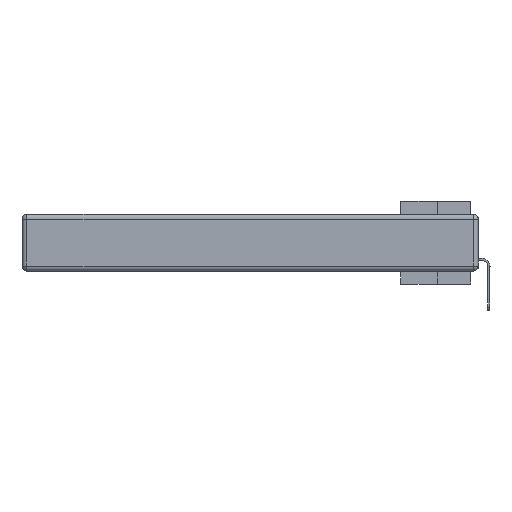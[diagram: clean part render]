
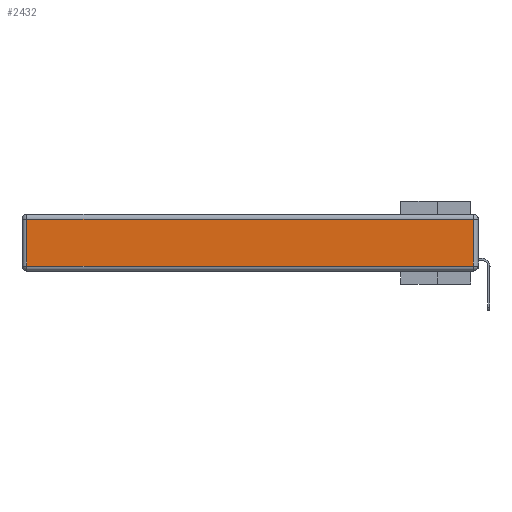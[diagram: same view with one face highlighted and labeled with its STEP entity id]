
A CAD part, left-side view. The second image highlights one B-rep face of the part: STEP entity #2432.
In plain terms, the highlighted planar face has unit normal (-1, 0, 0).
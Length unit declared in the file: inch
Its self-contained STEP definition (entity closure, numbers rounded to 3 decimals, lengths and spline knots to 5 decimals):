
#1082 = EDGE_CURVE ( 'NONE', #26887, #24364, #32122, .T. ) ;
#2432 = ADVANCED_FACE ( 'NONE', ( #31407 ), #2922, .T. ) ;
#2479 = EDGE_CURVE ( 'NONE', #24364, #10442, #26442, .T. ) ;
#2922 = PLANE ( 'NONE',  #15462 ) ;
#3279 = CARTESIAN_POINT ( 'NONE',  ( 0., 0.03, -0.03 ) ) ;
#4128 = CARTESIAN_POINT ( 'NONE',  ( 0., 0.03, -0.343 ) ) ;
#4857 = DIRECTION ( 'NONE',  ( 0., -1., 0. ) ) ;
#6007 = CARTESIAN_POINT ( 'NONE',  ( 0., 0.03, -0.313 ) ) ;
#6900 = LINE ( 'NONE', #17459, #11616 ) ;
#7398 = VECTOR ( 'NONE', #24774, 39.37008 ) ;
#7425 = EDGE_LOOP ( 'NONE', ( #19814, #25896, #20448, #9498 ) ) ;
#9498 = ORIENTED_EDGE ( 'NONE', *, *, #2479, .T. ) ;
#10442 = VERTEX_POINT ( 'NONE', #25561 ) ;
#10446 = DIRECTION ( 'NONE',  ( 0., 0., 1. ) ) ;
#10557 = VECTOR ( 'NONE', #15560, 39.37008 ) ;
#11421 = VERTEX_POINT ( 'NONE', #6007 ) ;
#11616 = VECTOR ( 'NONE', #4857, 39.37008 ) ;
#14531 = CARTESIAN_POINT ( 'NONE',  ( 0., 2.72, -0.03 ) ) ;
#15462 = AXIS2_PLACEMENT_3D ( 'NONE', #20674, #31083, #10446 ) ;
#15560 = DIRECTION ( 'NONE',  ( 0., 0., -1. ) ) ;
#17459 = CARTESIAN_POINT ( 'NONE',  ( 0., 0., -0.313 ) ) ;
#19814 = ORIENTED_EDGE ( 'NONE', *, *, #27907, .T. ) ;
#20448 = ORIENTED_EDGE ( 'NONE', *, *, #1082, .T. ) ;
#20674 = CARTESIAN_POINT ( 'NONE',  ( 0., 0., -0.343 ) ) ;
#24364 = VERTEX_POINT ( 'NONE', #14531 ) ;
#24774 = DIRECTION ( 'NONE',  ( 0., 1., 0. ) ) ;
#25561 = CARTESIAN_POINT ( 'NONE',  ( 0., 2.72, -0.313 ) ) ;
#25775 = CARTESIAN_POINT ( 'NONE',  ( 0., 2.72, -0.343 ) ) ;
#25896 = ORIENTED_EDGE ( 'NONE', *, *, #32437, .T. ) ;
#26442 = LINE ( 'NONE', #25775, #10557 ) ;
#26887 = VERTEX_POINT ( 'NONE', #3279 ) ;
#27652 = DIRECTION ( 'NONE',  ( 0., 0., 1. ) ) ;
#27907 = EDGE_CURVE ( 'NONE', #10442, #11421, #6900, .T. ) ;
#31083 = DIRECTION ( 'NONE',  ( -1., 0., 0. ) ) ;
#31407 = FACE_OUTER_BOUND ( 'NONE', #7425, .T. ) ;
#32122 = LINE ( 'NONE', #32289, #7398 ) ;
#32157 = VECTOR ( 'NONE', #27652, 39.37008 ) ;
#32289 = CARTESIAN_POINT ( 'NONE',  ( 0., 2.75, -0.03 ) ) ;
#32437 = EDGE_CURVE ( 'NONE', #11421, #26887, #32783, .T. ) ;
#32783 = LINE ( 'NONE', #4128, #32157 ) ;
